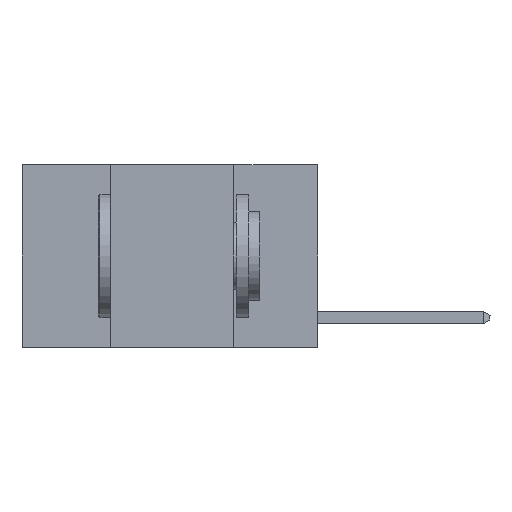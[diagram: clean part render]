
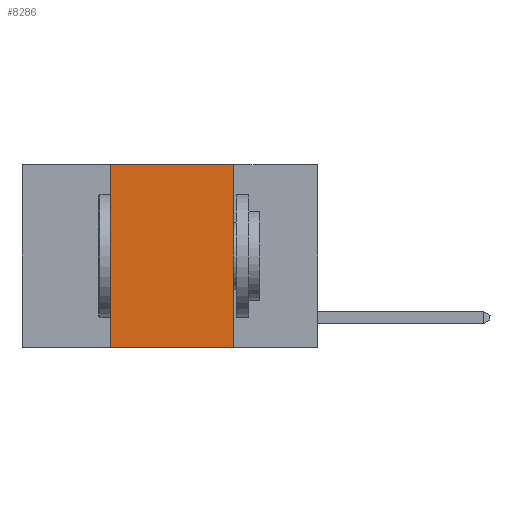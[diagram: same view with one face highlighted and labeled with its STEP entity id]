
A CAD part, left-side view. The second image highlights one B-rep face of the part: STEP entity #8286.
In plain terms, the highlighted planar face has unit normal (-1, 0, 0).
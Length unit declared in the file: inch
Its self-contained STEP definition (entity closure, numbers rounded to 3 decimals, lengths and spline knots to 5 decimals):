
#230 = VERTEX_POINT ( 'NONE', #3674 ) ;
#298 = AXIS2_PLACEMENT_3D ( 'NONE', #8763, #8688, #8614 ) ;
#938 = CARTESIAN_POINT ( 'NONE',  ( 0., 0.42, -0.37 ) ) ;
#1057 = FACE_OUTER_BOUND ( 'NONE', #4961, .T. ) ;
#1740 = VECTOR ( 'NONE', #5426, 39.37008 ) ;
#1793 = VERTEX_POINT ( 'NONE', #8757 ) ;
#1834 = VECTOR ( 'NONE', #5617, 39.37008 ) ;
#1890 = LINE ( 'NONE', #5505, #1834 ) ;
#2024 = LINE ( 'NONE', #5452, #1740 ) ;
#2076 = VECTOR ( 'NONE', #5769, 39.37008 ) ;
#2266 = LINE ( 'NONE', #5720, #2076 ) ;
#2432 = CARTESIAN_POINT ( 'NONE',  ( 0., 0.42, 0. ) ) ;
#3674 = CARTESIAN_POINT ( 'NONE',  ( 0., 0.17, 0. ) ) ;
#4961 = EDGE_LOOP ( 'NONE', ( #5217, #6952, #8335, #8474 ) ) ;
#5217 = ORIENTED_EDGE ( 'NONE', *, *, #6844, .F. ) ;
#5315 = VECTOR ( 'NONE', #8887, 39.37008 ) ;
#5426 = DIRECTION ( 'NONE',  ( 0., -1., 0. ) ) ;
#5452 = CARTESIAN_POINT ( 'NONE',  ( 0., 0.6, -0.37 ) ) ;
#5505 = CARTESIAN_POINT ( 'NONE',  ( 0., 0.42, 0. ) ) ;
#5509 = LINE ( 'NONE', #8867, #5315 ) ;
#5559 = PLANE ( 'NONE',  #298 ) ;
#5617 = DIRECTION ( 'NONE',  ( 0., 0., 1. ) ) ;
#5720 = CARTESIAN_POINT ( 'NONE',  ( 0., 0.17, 0. ) ) ;
#5769 = DIRECTION ( 'NONE',  ( 0., 0., -1. ) ) ;
#6632 = EDGE_CURVE ( 'NONE', #7136, #230, #5509, .T. ) ;
#6844 = EDGE_CURVE ( 'NONE', #230, #1793, #2266, .T. ) ;
#6851 = EDGE_CURVE ( 'NONE', #8723, #7136, #1890, .T. ) ;
#6859 = EDGE_CURVE ( 'NONE', #8723, #1793, #2024, .T. ) ;
#6952 = ORIENTED_EDGE ( 'NONE', *, *, #6632, .F. ) ;
#7136 = VERTEX_POINT ( 'NONE', #2432 ) ;
#8286 = ADVANCED_FACE ( 'NONE', ( #1057 ), #5559, .F. ) ;
#8335 = ORIENTED_EDGE ( 'NONE', *, *, #6851, .F. ) ;
#8474 = ORIENTED_EDGE ( 'NONE', *, *, #6859, .T. ) ;
#8614 = DIRECTION ( 'NONE',  ( 0., 0., -1. ) ) ;
#8688 = DIRECTION ( 'NONE',  ( 1., 0., 0. ) ) ;
#8723 = VERTEX_POINT ( 'NONE', #938 ) ;
#8757 = CARTESIAN_POINT ( 'NONE',  ( 0., 0.17, -0.37 ) ) ;
#8763 = CARTESIAN_POINT ( 'NONE',  ( 0., 0.6, 0. ) ) ;
#8867 = CARTESIAN_POINT ( 'NONE',  ( 0., 0.6, 0. ) ) ;
#8887 = DIRECTION ( 'NONE',  ( 0., -1., 0. ) ) ;
